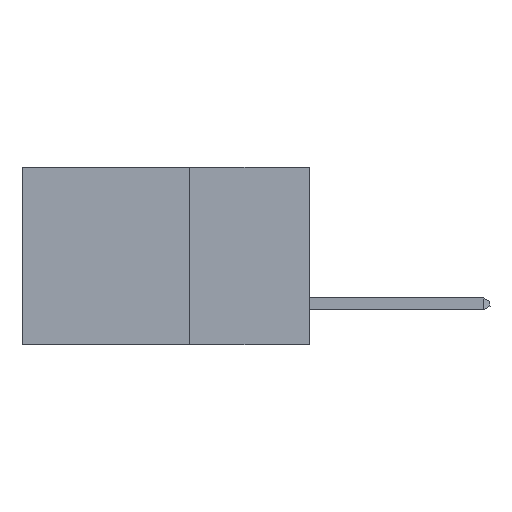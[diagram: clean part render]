
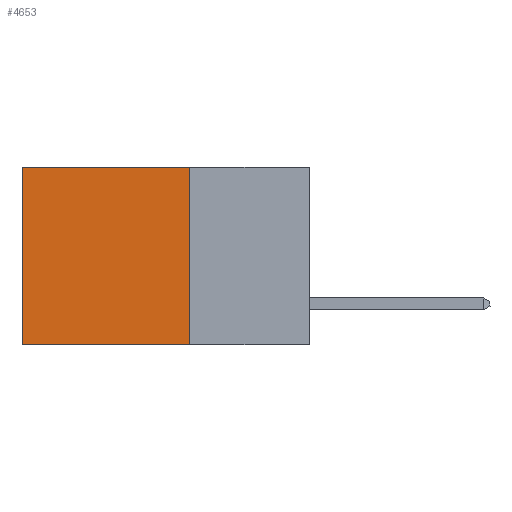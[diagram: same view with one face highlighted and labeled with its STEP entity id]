
A CAD part, left-side view. The second image highlights one B-rep face of the part: STEP entity #4653.
In plain terms, the highlighted planar face has unit normal (-1, 0, 0).
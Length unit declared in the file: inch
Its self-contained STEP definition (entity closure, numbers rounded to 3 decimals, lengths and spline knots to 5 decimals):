
#398 = CARTESIAN_POINT ( 'NONE',  ( 0.2875, 0.25, -0.37 ) ) ;
#1093 = CARTESIAN_POINT ( 'NONE',  ( 0.2875, 0.25, 0. ) ) ;
#1304 = DIRECTION ( 'NONE',  ( 0., 1., 0. ) ) ;
#1712 = LINE ( 'NONE', #398, #3791 ) ;
#2465 = CARTESIAN_POINT ( 'NONE',  ( 0.2875, 0.25, -0.37 ) ) ;
#2931 = CARTESIAN_POINT ( 'NONE',  ( 0.2875, 0.6, 0. ) ) ;
#3103 = LINE ( 'NONE', #1093, #5427 ) ;
#3631 = DIRECTION ( 'NONE',  ( 0., 1., 0. ) ) ;
#3663 = CARTESIAN_POINT ( 'NONE',  ( 0.2875, 0.6, 0. ) ) ;
#3750 = LINE ( 'NONE', #8803, #8064 ) ;
#3791 = VECTOR ( 'NONE', #1304, 39.37008 ) ;
#3827 = DIRECTION ( 'NONE',  ( 0., 0., -1. ) ) ;
#4369 = CARTESIAN_POINT ( 'NONE',  ( 0.2875, 0.25, 0. ) ) ;
#4444 = EDGE_CURVE ( 'NONE', #10472, #7649, #3103, .T. ) ;
#4646 = EDGE_CURVE ( 'NONE', #7649, #6869, #1712, .T. ) ;
#4653 = ADVANCED_FACE ( 'NONE', ( #7837 ), #7502, .F. ) ;
#4928 = LINE ( 'NONE', #2931, #11050 ) ;
#4938 = DIRECTION ( 'NONE',  ( 1., 0., 0. ) ) ;
#5427 = VECTOR ( 'NONE', #8983, 39.37008 ) ;
#5759 = EDGE_LOOP ( 'NONE', ( #8316, #8570, #8635, #8865 ) ) ;
#6869 = VERTEX_POINT ( 'NONE', #10879 ) ;
#7180 = EDGE_CURVE ( 'NONE', #10472, #8400, #3750, .T. ) ;
#7502 = PLANE ( 'NONE',  #9700 ) ;
#7649 = VERTEX_POINT ( 'NONE', #2465 ) ;
#7837 = FACE_OUTER_BOUND ( 'NONE', #5759, .T. ) ;
#8064 = VECTOR ( 'NONE', #3631, 39.37008 ) ;
#8316 = ORIENTED_EDGE ( 'NONE', *, *, #10005, .T. ) ;
#8400 = VERTEX_POINT ( 'NONE', #3663 ) ;
#8570 = ORIENTED_EDGE ( 'NONE', *, *, #4646, .F. ) ;
#8635 = ORIENTED_EDGE ( 'NONE', *, *, #4444, .F. ) ;
#8803 = CARTESIAN_POINT ( 'NONE',  ( 0.2875, 0.25, 0. ) ) ;
#8865 = ORIENTED_EDGE ( 'NONE', *, *, #7180, .T. ) ;
#8983 = DIRECTION ( 'NONE',  ( 0., 0., -1. ) ) ;
#9700 = AXIS2_PLACEMENT_3D ( 'NONE', #10027, #4938, #10800 ) ;
#10005 = EDGE_CURVE ( 'NONE', #8400, #6869, #4928, .T. ) ;
#10027 = CARTESIAN_POINT ( 'NONE',  ( 0.2875, 0.25, 0. ) ) ;
#10472 = VERTEX_POINT ( 'NONE', #4369 ) ;
#10800 = DIRECTION ( 'NONE',  ( 0., 0., -1. ) ) ;
#10879 = CARTESIAN_POINT ( 'NONE',  ( 0.2875, 0.6, -0.37 ) ) ;
#11050 = VECTOR ( 'NONE', #3827, 39.37008 ) ;
